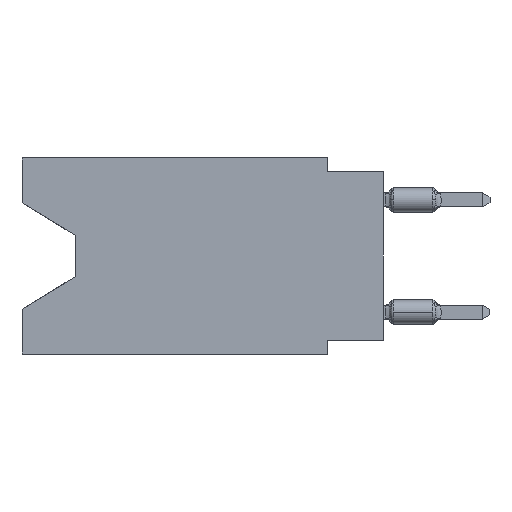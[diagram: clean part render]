
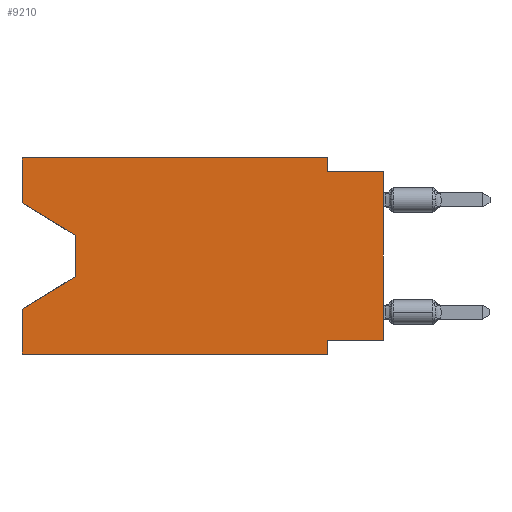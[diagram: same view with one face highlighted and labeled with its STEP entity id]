
A CAD part, left-side view. The second image highlights one B-rep face of the part: STEP entity #9210.
In plain terms, the highlighted planar face has unit normal (-1, 0, 0).
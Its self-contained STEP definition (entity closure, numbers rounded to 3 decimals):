
#184 = VECTOR ( 'NONE', #18168, 1000. ) ;
#256 = DIRECTION ( 'NONE',  ( 0., 0.855, -0.519 ) ) ;
#331 = DIRECTION ( 'NONE',  ( 0., 0., 1. ) ) ;
#470 = CARTESIAN_POINT ( 'NONE',  ( 0., 16.383, -2.038 ) ) ;
#478 = VECTOR ( 'NONE', #14697, 1000. ) ;
#690 = VERTEX_POINT ( 'NONE', #10330 ) ;
#717 = ORIENTED_EDGE ( 'NONE', *, *, #3394, .F. ) ;
#844 = CARTESIAN_POINT ( 'NONE',  ( 0., 2.54, -8.89 ) ) ;
#992 = DIRECTION ( 'NONE',  ( 1., 0., 0. ) ) ;
#1226 = CARTESIAN_POINT ( 'NONE',  ( 0., 2.54, -0.635 ) ) ;
#1342 = VERTEX_POINT ( 'NONE', #8437 ) ;
#1563 = LINE ( 'NONE', #18681, #13051 ) ;
#1687 = CARTESIAN_POINT ( 'NONE',  ( 0., 0., -8.255 ) ) ;
#1903 = CARTESIAN_POINT ( 'NONE',  ( 0., 0., 0. ) ) ;
#2121 = DIRECTION ( 'NONE',  ( 0., 1., 0. ) ) ;
#2127 = CARTESIAN_POINT ( 'NONE',  ( 0., 2.54, 0. ) ) ;
#2196 = EDGE_CURVE ( 'NONE', #19269, #3929, #6566, .T. ) ;
#2358 = DIRECTION ( 'NONE',  ( 0., -1., 0. ) ) ;
#2443 = VECTOR ( 'NONE', #3742, 1000. ) ;
#2993 = CARTESIAN_POINT ( 'NONE',  ( 0., 16.383, 0. ) ) ;
#3107 = VECTOR ( 'NONE', #331, 1000. ) ;
#3394 = EDGE_CURVE ( 'NONE', #3929, #13272, #17717, .T. ) ;
#3546 = DIRECTION ( 'NONE',  ( 0., 0., -1. ) ) ;
#3696 = EDGE_CURVE ( 'NONE', #17372, #11481, #6014, .T. ) ;
#3742 = DIRECTION ( 'NONE',  ( 0., -1., 0. ) ) ;
#3929 = VERTEX_POINT ( 'NONE', #1226 ) ;
#3967 = ORIENTED_EDGE ( 'NONE', *, *, #11871, .F. ) ;
#4012 = DIRECTION ( 'NONE',  ( 0., 0., -1. ) ) ;
#4061 = VECTOR ( 'NONE', #3546, 1000. ) ;
#4187 = CARTESIAN_POINT ( 'NONE',  ( 0., 0., -0.635 ) ) ;
#4302 = CARTESIAN_POINT ( 'NONE',  ( 0., 13.97, -5.385 ) ) ;
#4443 = CARTESIAN_POINT ( 'NONE',  ( 0., 16.383, -2.038 ) ) ;
#4513 = ORIENTED_EDGE ( 'NONE', *, *, #17297, .T. ) ;
#4526 = CARTESIAN_POINT ( 'NONE',  ( 0., 16.383, -6.852 ) ) ;
#5257 = CARTESIAN_POINT ( 'NONE',  ( 0., 0., -0.635 ) ) ;
#5538 = EDGE_CURVE ( 'NONE', #11481, #19269, #12230, .T. ) ;
#5564 = CARTESIAN_POINT ( 'NONE',  ( 0., 2.54, -8.89 ) ) ;
#5625 = EDGE_CURVE ( 'NONE', #17372, #12608, #16674, .T. ) ;
#6014 = LINE ( 'NONE', #2993, #184 ) ;
#6183 = ORIENTED_EDGE ( 'NONE', *, *, #2196, .F. ) ;
#6375 = VECTOR ( 'NONE', #16972, 1000. ) ;
#6386 = CARTESIAN_POINT ( 'NONE',  ( 0., 16.383, 0. ) ) ;
#6566 = LINE ( 'NONE', #2127, #4061 ) ;
#6704 = ORIENTED_EDGE ( 'NONE', *, *, #5538, .F. ) ;
#7177 = LINE ( 'NONE', #19254, #12143 ) ;
#8078 = VERTEX_POINT ( 'NONE', #4526 ) ;
#8386 = LINE ( 'NONE', #9807, #10490 ) ;
#8437 = CARTESIAN_POINT ( 'NONE',  ( 0., 2.54, -8.255 ) ) ;
#8790 = DIRECTION ( 'NONE',  ( 0., 0., -1. ) ) ;
#9210 = ADVANCED_FACE ( 'NONE', ( #10016 ), #17703, .F. ) ;
#9807 = CARTESIAN_POINT ( 'NONE',  ( 0., 0., -8.255 ) ) ;
#9882 = LINE ( 'NONE', #12268, #3107 ) ;
#10016 = FACE_OUTER_BOUND ( 'NONE', #13406, .T. ) ;
#10330 = CARTESIAN_POINT ( 'NONE',  ( 0., 16.383, -8.89 ) ) ;
#10490 = VECTOR ( 'NONE', #2121, 1000. ) ;
#10612 = DIRECTION ( 'NONE',  ( 0., -0.855, -0.519 ) ) ;
#11296 = LINE ( 'NONE', #1903, #16029 ) ;
#11481 = VERTEX_POINT ( 'NONE', #6386 ) ;
#11678 = EDGE_CURVE ( 'NONE', #12608, #18781, #17817, .T. ) ;
#11871 = EDGE_CURVE ( 'NONE', #1342, #17785, #13280, .T. ) ;
#12143 = VECTOR ( 'NONE', #2358, 1000. ) ;
#12230 = LINE ( 'NONE', #18199, #6375 ) ;
#12233 = EDGE_CURVE ( 'NONE', #19397, #1342, #8386, .T. ) ;
#12268 = CARTESIAN_POINT ( 'NONE',  ( 0., 16.383, 0. ) ) ;
#12608 = VERTEX_POINT ( 'NONE', #14237 ) ;
#13051 = VECTOR ( 'NONE', #256, 1000. ) ;
#13251 = CARTESIAN_POINT ( 'NONE',  ( 0., 2.54, 0. ) ) ;
#13272 = VERTEX_POINT ( 'NONE', #4187 ) ;
#13280 = LINE ( 'NONE', #844, #478 ) ;
#13367 = ORIENTED_EDGE ( 'NONE', *, *, #13579, .T. ) ;
#13406 = EDGE_LOOP ( 'NONE', ( #18471, #13909, #18541, #15623, #13367, #3967, #18802, #4513, #717, #6183, #6704, #15462 ) ) ;
#13579 = EDGE_CURVE ( 'NONE', #690, #17785, #7177, .T. ) ;
#13909 = ORIENTED_EDGE ( 'NONE', *, *, #11678, .T. ) ;
#14233 = DIRECTION ( 'NONE',  ( 0., 0., 1. ) ) ;
#14237 = CARTESIAN_POINT ( 'NONE',  ( 0., 13.97, -3.505 ) ) ;
#14697 = DIRECTION ( 'NONE',  ( 0., 0., -1. ) ) ;
#15107 = AXIS2_PLACEMENT_3D ( 'NONE', #19425, #992, #4012 ) ;
#15462 = ORIENTED_EDGE ( 'NONE', *, *, #3696, .F. ) ;
#15623 = ORIENTED_EDGE ( 'NONE', *, *, #17511, .F. ) ;
#15904 = EDGE_CURVE ( 'NONE', #18781, #8078, #1563, .T. ) ;
#16029 = VECTOR ( 'NONE', #14233, 1000. ) ;
#16396 = CARTESIAN_POINT ( 'NONE',  ( 0., 13.97, -3.505 ) ) ;
#16674 = LINE ( 'NONE', #4443, #17376 ) ;
#16972 = DIRECTION ( 'NONE',  ( 0., -1., 0. ) ) ;
#17297 = EDGE_CURVE ( 'NONE', #19397, #13272, #11296, .T. ) ;
#17372 = VERTEX_POINT ( 'NONE', #470 ) ;
#17376 = VECTOR ( 'NONE', #10612, 1000. ) ;
#17511 = EDGE_CURVE ( 'NONE', #690, #8078, #9882, .T. ) ;
#17703 = PLANE ( 'NONE',  #15107 ) ;
#17717 = LINE ( 'NONE', #5257, #2443 ) ;
#17785 = VERTEX_POINT ( 'NONE', #5564 ) ;
#17817 = LINE ( 'NONE', #16396, #18240 ) ;
#18168 = DIRECTION ( 'NONE',  ( 0., 0., 1. ) ) ;
#18199 = CARTESIAN_POINT ( 'NONE',  ( 0., 16.383, 0. ) ) ;
#18240 = VECTOR ( 'NONE', #8790, 1000. ) ;
#18471 = ORIENTED_EDGE ( 'NONE', *, *, #5625, .T. ) ;
#18541 = ORIENTED_EDGE ( 'NONE', *, *, #15904, .T. ) ;
#18681 = CARTESIAN_POINT ( 'NONE',  ( 0., 13.97, -5.385 ) ) ;
#18781 = VERTEX_POINT ( 'NONE', #4302 ) ;
#18802 = ORIENTED_EDGE ( 'NONE', *, *, #12233, .F. ) ;
#19254 = CARTESIAN_POINT ( 'NONE',  ( 0., 16.383, -8.89 ) ) ;
#19269 = VERTEX_POINT ( 'NONE', #13251 ) ;
#19397 = VERTEX_POINT ( 'NONE', #1687 ) ;
#19425 = CARTESIAN_POINT ( 'NONE',  ( 0., 16.383, 0. ) ) ;
